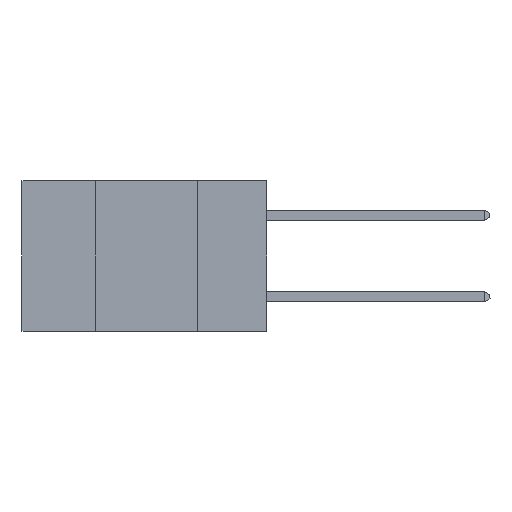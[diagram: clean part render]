
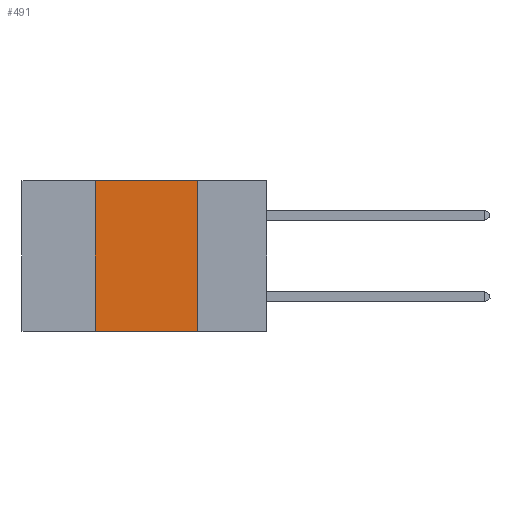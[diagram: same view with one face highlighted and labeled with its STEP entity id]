
A CAD part, left-side view. The second image highlights one B-rep face of the part: STEP entity #491.
In plain terms, the highlighted planar face has unit normal (-1, 0, 0).
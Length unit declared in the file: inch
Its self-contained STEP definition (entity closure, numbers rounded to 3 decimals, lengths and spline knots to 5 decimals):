
#63 = AXIS2_PLACEMENT_3D ( 'NONE', #3392, #2412, #4746 ) ;
#312 = VERTEX_POINT ( 'NONE', #5164 ) ;
#491 = ADVANCED_FACE ( 'NONE', ( #6752 ), #1674, .F. ) ;
#1039 = EDGE_CURVE ( 'NONE', #312, #7013, #7535, .T. ) ;
#1061 = DIRECTION ( 'NONE',  ( 0., 0., 1. ) ) ;
#1674 = PLANE ( 'NONE',  #63 ) ;
#2130 = VERTEX_POINT ( 'NONE', #8459 ) ;
#2355 = VERTEX_POINT ( 'NONE', #4282 ) ;
#2412 = DIRECTION ( 'NONE',  ( 1., 0., 0. ) ) ;
#2445 = ORIENTED_EDGE ( 'NONE', *, *, #3979, .F. ) ;
#2621 = ORIENTED_EDGE ( 'NONE', *, *, #1039, .F. ) ;
#2819 = LINE ( 'NONE', #3024, #6592 ) ;
#2973 = CARTESIAN_POINT ( 'NONE',  ( 0., 0.6, 0. ) ) ;
#3024 = CARTESIAN_POINT ( 'NONE',  ( 0., 0.6, -0.37 ) ) ;
#3080 = ORIENTED_EDGE ( 'NONE', *, *, #5990, .T. ) ;
#3190 = LINE ( 'NONE', #5013, #8933 ) ;
#3218 = DIRECTION ( 'NONE',  ( 0., -1., 0. ) ) ;
#3392 = CARTESIAN_POINT ( 'NONE',  ( 0., 0.6, 0. ) ) ;
#3979 = EDGE_CURVE ( 'NONE', #7013, #2130, #7532, .T. ) ;
#4282 = CARTESIAN_POINT ( 'NONE',  ( 0., 0.17, -0.37 ) ) ;
#4511 = EDGE_CURVE ( 'NONE', #2130, #2355, #3190, .T. ) ;
#4746 = DIRECTION ( 'NONE',  ( 0., 0., -1. ) ) ;
#4772 = CARTESIAN_POINT ( 'NONE',  ( 0., 0.42, 0. ) ) ;
#4831 = VECTOR ( 'NONE', #3218, 39.37008 ) ;
#5013 = CARTESIAN_POINT ( 'NONE',  ( 0., 0.17, 0. ) ) ;
#5164 = CARTESIAN_POINT ( 'NONE',  ( 0., 0.42, -0.37 ) ) ;
#5643 = DIRECTION ( 'NONE',  ( 0., 0., -1. ) ) ;
#5959 = DIRECTION ( 'NONE',  ( 0., -1., 0. ) ) ;
#5990 = EDGE_CURVE ( 'NONE', #312, #2355, #2819, .T. ) ;
#6122 = VECTOR ( 'NONE', #1061, 39.37008 ) ;
#6508 = ORIENTED_EDGE ( 'NONE', *, *, #4511, .F. ) ;
#6592 = VECTOR ( 'NONE', #5959, 39.37008 ) ;
#6752 = FACE_OUTER_BOUND ( 'NONE', #7711, .T. ) ;
#7013 = VERTEX_POINT ( 'NONE', #7741 ) ;
#7532 = LINE ( 'NONE', #2973, #4831 ) ;
#7535 = LINE ( 'NONE', #4772, #6122 ) ;
#7711 = EDGE_LOOP ( 'NONE', ( #6508, #2445, #2621, #3080 ) ) ;
#7741 = CARTESIAN_POINT ( 'NONE',  ( 0., 0.42, 0. ) ) ;
#8459 = CARTESIAN_POINT ( 'NONE',  ( 0., 0.17, 0. ) ) ;
#8933 = VECTOR ( 'NONE', #5643, 39.37008 ) ;
